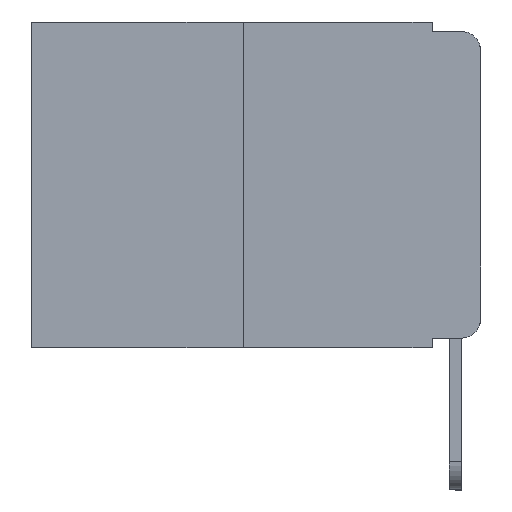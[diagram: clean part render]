
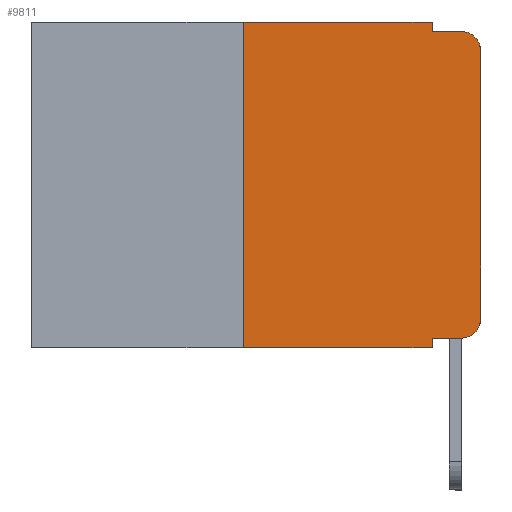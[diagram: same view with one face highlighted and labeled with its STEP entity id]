
A CAD part, left-side view. The second image highlights one B-rep face of the part: STEP entity #9811.
In plain terms, the highlighted planar face has unit normal (-1, 0, 0).
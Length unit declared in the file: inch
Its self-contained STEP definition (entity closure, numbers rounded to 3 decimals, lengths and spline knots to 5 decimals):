
#127 = EDGE_CURVE ( 'NONE', #1303, #6730, #11726, .T. ) ;
#364 = CARTESIAN_POINT ( 'NONE',  ( 0., 0., -0.03 ) ) ;
#510 = LINE ( 'NONE', #7536, #3848 ) ;
#530 = CIRCLE ( 'NONE', #13709, 0.02 ) ;
#537 = ORIENTED_EDGE ( 'NONE', *, *, #3766, .T. ) ;
#786 = DIRECTION ( 'NONE',  ( -1., 0., 0. ) ) ;
#926 = CARTESIAN_POINT ( 'NONE',  ( 0., 0.02, -0.01 ) ) ;
#994 = CARTESIAN_POINT ( 'NONE',  ( 0., 0.051, -0.01 ) ) ;
#1303 = VERTEX_POINT ( 'NONE', #7004 ) ;
#2144 = VERTEX_POINT ( 'NONE', #10523 ) ;
#2228 = ORIENTED_EDGE ( 'NONE', *, *, #9728, .F. ) ;
#2406 = VECTOR ( 'NONE', #10831, 39.37008 ) ;
#2414 = VERTEX_POINT ( 'NONE', #994 ) ;
#2503 = LINE ( 'NONE', #15310, #12369 ) ;
#2610 = VERTEX_POINT ( 'NONE', #6009 ) ;
#2623 = EDGE_CURVE ( 'NONE', #11521, #2414, #2503, .T. ) ;
#2771 = AXIS2_PLACEMENT_3D ( 'NONE', #9142, #5489, #4485 ) ;
#3071 = CARTESIAN_POINT ( 'NONE',  ( 0., 0.473, 0. ) ) ;
#3088 = AXIS2_PLACEMENT_3D ( 'NONE', #3071, #13851, #15306 ) ;
#3254 = EDGE_CURVE ( 'NONE', #11638, #5249, #13899, .T. ) ;
#3332 = EDGE_CURVE ( 'NONE', #2610, #11638, #12086, .T. ) ;
#3486 = ORIENTED_EDGE ( 'NONE', *, *, #127, .T. ) ;
#3766 = EDGE_CURVE ( 'NONE', #2144, #5276, #13226, .T. ) ;
#3848 = VECTOR ( 'NONE', #4131, 39.37008 ) ;
#4131 = DIRECTION ( 'NONE',  ( 0., -1., 0. ) ) ;
#4159 = FACE_OUTER_BOUND ( 'NONE', #12984, .T. ) ;
#4485 = DIRECTION ( 'NONE',  ( 0., 0., -1. ) ) ;
#4539 = VECTOR ( 'NONE', #11291, 39.37008 ) ;
#5249 = VERTEX_POINT ( 'NONE', #926 ) ;
#5276 = VERTEX_POINT ( 'NONE', #15139 ) ;
#5315 = DIRECTION ( 'NONE',  ( 0., 0., 1. ) ) ;
#5418 = EDGE_CURVE ( 'NONE', #1303, #5276, #7323, .T. ) ;
#5489 = DIRECTION ( 'NONE',  ( -1., 0., 0. ) ) ;
#5887 = CARTESIAN_POINT ( 'NONE',  ( 0., 0., 0. ) ) ;
#6009 = CARTESIAN_POINT ( 'NONE',  ( 0., 0., -0.313 ) ) ;
#6730 = VERTEX_POINT ( 'NONE', #14561 ) ;
#7004 = CARTESIAN_POINT ( 'NONE',  ( 0., 0.051, -0.333 ) ) ;
#7260 = DIRECTION ( 'NONE',  ( 0., 0., -1. ) ) ;
#7323 = LINE ( 'NONE', #9579, #15088 ) ;
#7536 = CARTESIAN_POINT ( 'NONE',  ( 0., 0.473, 0. ) ) ;
#7546 = VERTEX_POINT ( 'NONE', #13192 ) ;
#8254 = EDGE_CURVE ( 'NONE', #6730, #2610, #530, .T. ) ;
#8527 = EDGE_CURVE ( 'NONE', #2414, #5249, #12453, .T. ) ;
#9142 = CARTESIAN_POINT ( 'NONE',  ( 0., 0.02, -0.03 ) ) ;
#9444 = CARTESIAN_POINT ( 'NONE',  ( 0., 0.473, -0.343 ) ) ;
#9579 = CARTESIAN_POINT ( 'NONE',  ( 0., 0.051, 0. ) ) ;
#9629 = ORIENTED_EDGE ( 'NONE', *, *, #3254, .T. ) ;
#9728 = EDGE_CURVE ( 'NONE', #2144, #7546, #12542, .T. ) ;
#9811 = ADVANCED_FACE ( 'NONE', ( #4159 ), #13619, .F. ) ;
#10321 = CARTESIAN_POINT ( 'NONE',  ( 0., 0.051, -0.333 ) ) ;
#10339 = CARTESIAN_POINT ( 'NONE',  ( 0., 0.051, 0. ) ) ;
#10360 = ORIENTED_EDGE ( 'NONE', *, *, #11723, .F. ) ;
#10523 = CARTESIAN_POINT ( 'NONE',  ( 0., 0.25, -0.343 ) ) ;
#10831 = DIRECTION ( 'NONE',  ( 0., -1., 0. ) ) ;
#11291 = DIRECTION ( 'NONE',  ( 0., -1., 0. ) ) ;
#11375 = ORIENTED_EDGE ( 'NONE', *, *, #3332, .T. ) ;
#11446 = ORIENTED_EDGE ( 'NONE', *, *, #8254, .T. ) ;
#11479 = DIRECTION ( 'NONE',  ( 0., -1., 0. ) ) ;
#11490 = ORIENTED_EDGE ( 'NONE', *, *, #2623, .F. ) ;
#11521 = VERTEX_POINT ( 'NONE', #10339 ) ;
#11638 = VERTEX_POINT ( 'NONE', #364 ) ;
#11723 = EDGE_CURVE ( 'NONE', #7546, #11521, #510, .T. ) ;
#11726 = LINE ( 'NONE', #10321, #14135 ) ;
#12086 = LINE ( 'NONE', #5887, #14633 ) ;
#12369 = VECTOR ( 'NONE', #7260, 39.37008 ) ;
#12370 = CARTESIAN_POINT ( 'NONE',  ( 0., 0.051, -0.01 ) ) ;
#12375 = CARTESIAN_POINT ( 'NONE',  ( 0., 0.25, 0. ) ) ;
#12453 = LINE ( 'NONE', #12370, #4539 ) ;
#12542 = LINE ( 'NONE', #12375, #15207 ) ;
#12934 = DIRECTION ( 'NONE',  ( 0., 0., -1. ) ) ;
#12984 = EDGE_LOOP ( 'NONE', ( #11375, #9629, #13673, #11490, #10360, #2228, #537, #14898, #3486, #11446 ) ) ;
#13165 = DIRECTION ( 'NONE',  ( 0., 0., 1. ) ) ;
#13192 = CARTESIAN_POINT ( 'NONE',  ( 0., 0.25, 0. ) ) ;
#13226 = LINE ( 'NONE', #9444, #2406 ) ;
#13619 = PLANE ( 'NONE',  #3088 ) ;
#13673 = ORIENTED_EDGE ( 'NONE', *, *, #8527, .F. ) ;
#13709 = AXIS2_PLACEMENT_3D ( 'NONE', #15240, #786, #12934 ) ;
#13851 = DIRECTION ( 'NONE',  ( 1., 0., 0. ) ) ;
#13899 = CIRCLE ( 'NONE', #2771, 0.02 ) ;
#14135 = VECTOR ( 'NONE', #11479, 39.37008 ) ;
#14147 = DIRECTION ( 'NONE',  ( 0., 0., -1. ) ) ;
#14561 = CARTESIAN_POINT ( 'NONE',  ( 0., 0.02, -0.333 ) ) ;
#14633 = VECTOR ( 'NONE', #13165, 39.37008 ) ;
#14898 = ORIENTED_EDGE ( 'NONE', *, *, #5418, .F. ) ;
#15088 = VECTOR ( 'NONE', #14147, 39.37008 ) ;
#15139 = CARTESIAN_POINT ( 'NONE',  ( 0., 0.051, -0.343 ) ) ;
#15207 = VECTOR ( 'NONE', #5315, 39.37008 ) ;
#15240 = CARTESIAN_POINT ( 'NONE',  ( 0., 0.02, -0.313 ) ) ;
#15306 = DIRECTION ( 'NONE',  ( 0., 0., -1. ) ) ;
#15310 = CARTESIAN_POINT ( 'NONE',  ( 0., 0.051, 0. ) ) ;
